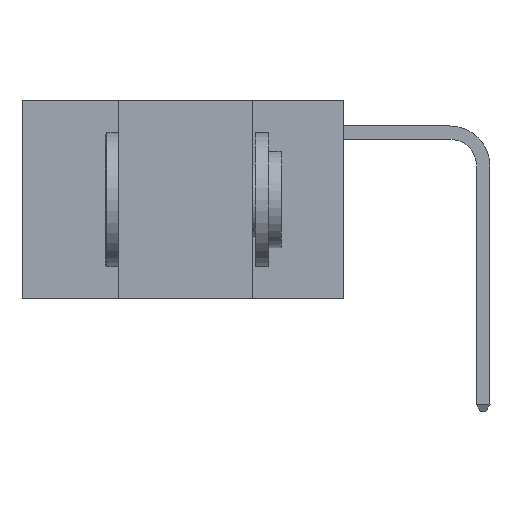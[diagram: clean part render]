
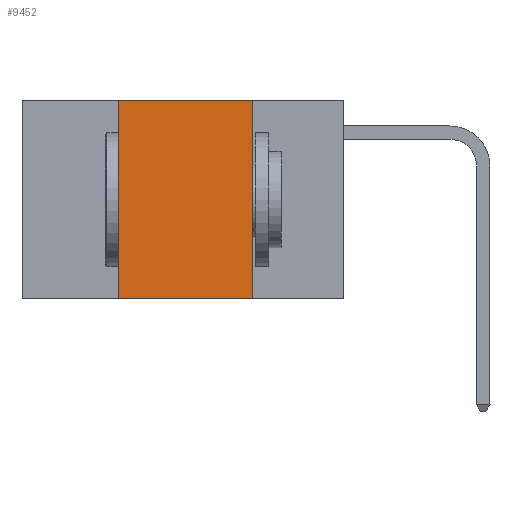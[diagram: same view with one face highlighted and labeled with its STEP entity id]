
A CAD part, left-side view. The second image highlights one B-rep face of the part: STEP entity #9452.
In plain terms, the highlighted planar face has unit normal (-1, 0, 0).
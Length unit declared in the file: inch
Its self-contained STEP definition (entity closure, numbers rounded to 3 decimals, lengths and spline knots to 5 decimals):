
#103 = ORIENTED_EDGE ( 'NONE', *, *, #4582, .F. ) ;
#135 = EDGE_CURVE ( 'NONE', #6755, #6966, #9033, .T. ) ;
#568 = LINE ( 'NONE', #6260, #2362 ) ;
#804 = FACE_OUTER_BOUND ( 'NONE', #9150, .T. ) ;
#1471 = CARTESIAN_POINT ( 'NONE',  ( 0., 0.6, -0.37 ) ) ;
#2362 = VECTOR ( 'NONE', #9260, 39.37008 ) ;
#2555 = CARTESIAN_POINT ( 'NONE',  ( 0., 0.6, 0. ) ) ;
#2920 = DIRECTION ( 'NONE',  ( 0., -1., 0. ) ) ;
#2931 = VERTEX_POINT ( 'NONE', #8648 ) ;
#3536 = CARTESIAN_POINT ( 'NONE',  ( 0., 0.17, 0. ) ) ;
#3807 = CARTESIAN_POINT ( 'NONE',  ( 0., 0.6, 0. ) ) ;
#4532 = ORIENTED_EDGE ( 'NONE', *, *, #8362, .T. ) ;
#4582 = EDGE_CURVE ( 'NONE', #2931, #6493, #568, .T. ) ;
#4611 = PLANE ( 'NONE',  #8979 ) ;
#4800 = CARTESIAN_POINT ( 'NONE',  ( 0., 0.17, 0. ) ) ;
#4851 = LINE ( 'NONE', #2555, #5795 ) ;
#5015 = DIRECTION ( 'NONE',  ( 0., -1., 0. ) ) ;
#5359 = ORIENTED_EDGE ( 'NONE', *, *, #135, .F. ) ;
#5503 = DIRECTION ( 'NONE',  ( 0., 0., -1. ) ) ;
#5795 = VECTOR ( 'NONE', #5015, 39.37008 ) ;
#6260 = CARTESIAN_POINT ( 'NONE',  ( 0., 0.42, 0. ) ) ;
#6493 = VERTEX_POINT ( 'NONE', #7174 ) ;
#6697 = DIRECTION ( 'NONE',  ( 1., 0., 0. ) ) ;
#6755 = VERTEX_POINT ( 'NONE', #3536 ) ;
#6843 = DIRECTION ( 'NONE',  ( 0., 0., -1. ) ) ;
#6881 = VECTOR ( 'NONE', #2920, 39.37008 ) ;
#6966 = VERTEX_POINT ( 'NONE', #8249 ) ;
#7174 = CARTESIAN_POINT ( 'NONE',  ( 0., 0.42, 0. ) ) ;
#8249 = CARTESIAN_POINT ( 'NONE',  ( 0., 0.17, -0.37 ) ) ;
#8362 = EDGE_CURVE ( 'NONE', #2931, #6966, #9744, .T. ) ;
#8429 = EDGE_CURVE ( 'NONE', #6493, #6755, #4851, .T. ) ;
#8648 = CARTESIAN_POINT ( 'NONE',  ( 0., 0.42, -0.37 ) ) ;
#8876 = VECTOR ( 'NONE', #5503, 39.37008 ) ;
#8979 = AXIS2_PLACEMENT_3D ( 'NONE', #3807, #6697, #6843 ) ;
#9033 = LINE ( 'NONE', #4800, #8876 ) ;
#9150 = EDGE_LOOP ( 'NONE', ( #5359, #9427, #103, #4532 ) ) ;
#9260 = DIRECTION ( 'NONE',  ( 0., 0., 1. ) ) ;
#9427 = ORIENTED_EDGE ( 'NONE', *, *, #8429, .F. ) ;
#9452 = ADVANCED_FACE ( 'NONE', ( #804 ), #4611, .F. ) ;
#9744 = LINE ( 'NONE', #1471, #6881 ) ;
